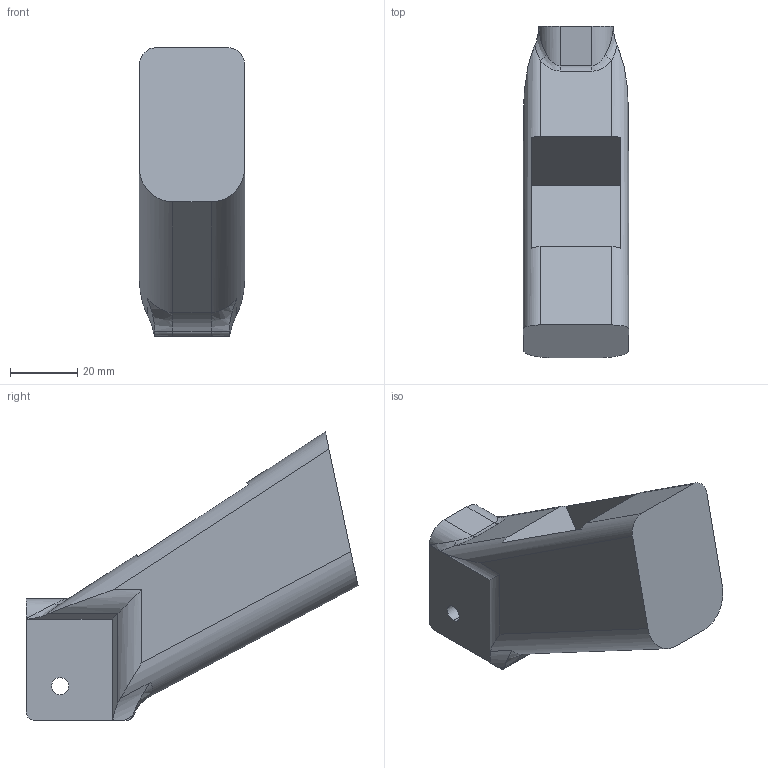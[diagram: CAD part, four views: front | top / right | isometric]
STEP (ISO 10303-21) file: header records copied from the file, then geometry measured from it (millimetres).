
FILE_DESCRIPTION (( 'STEP AP214' ), '1' );
FILE_NAME ('GripRemodeled.STEP', '2013-06-07T17:15:57', ( 'Asher' ), ( '' ), 'SwSTEP 2.0', 'SolidWorks 2013', '' );
FILE_SCHEMA (( 'AUTOMOTIVE_DESIGN' ));
Length unit declared in the file: inch
Products named in the file (1): GripRemodeled
Bounding box: 31.4 x 99.03 x 86.05 mm (x, y, z)
Volume: 86655.3 mm3; surface area: 20691.6 mm2
Topology: 1 solids, 1 shells, 56 faces, 152 edges, 98 vertices
Faces by surface type: plane 27, cylinder 21, bspline 8
Entity records: 2174 total; most frequent: CARTESIAN_POINT 829, ORIENTED_EDGE 304, DIRECTION 232, EDGE_CURVE 152, VERTEX_POINT 98, LINE 82, VECTOR 82, AXIS2_PLACEMENT_3D 75
